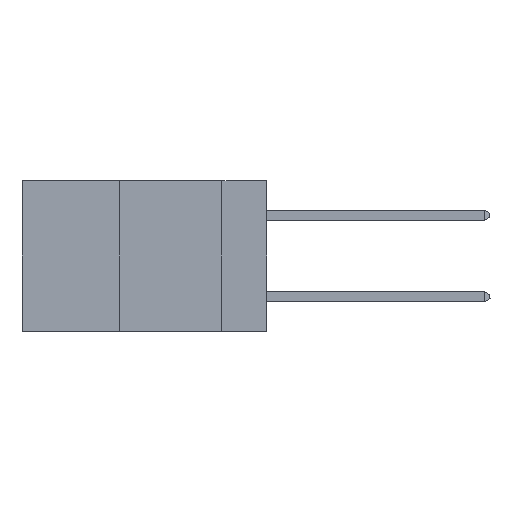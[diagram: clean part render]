
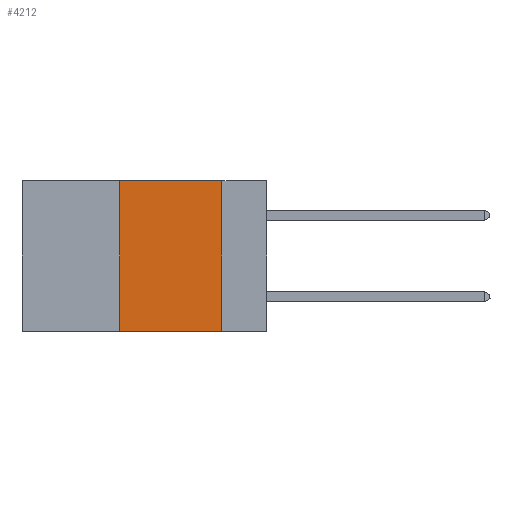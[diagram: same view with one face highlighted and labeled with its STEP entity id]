
A CAD part, left-side view. The second image highlights one B-rep face of the part: STEP entity #4212.
In plain terms, the highlighted planar face has unit normal (-1, 0, 0).
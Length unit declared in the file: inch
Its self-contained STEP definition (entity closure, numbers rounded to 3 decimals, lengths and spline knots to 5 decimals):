
#43 = DIRECTION ( 'NONE',  ( 0., 0., -1. ) ) ;
#694 = EDGE_CURVE ( 'NONE', #19665, #8763, #22387, .T. ) ;
#1122 = EDGE_LOOP ( 'NONE', ( #20354, #18112, #22234, #12950 ) ) ;
#1614 = VECTOR ( 'NONE', #10690, 39.37008 ) ;
#1922 = AXIS2_PLACEMENT_3D ( 'NONE', #17055, #19827, #19886 ) ;
#2214 = DIRECTION ( 'NONE',  ( 0., -1., 0. ) ) ;
#2495 = LINE ( 'NONE', #20569, #10209 ) ;
#2637 = VECTOR ( 'NONE', #43, 39.37008 ) ;
#4154 = EDGE_CURVE ( 'NONE', #19665, #20571, #2495, .T. ) ;
#4212 = ADVANCED_FACE ( 'NONE', ( #9643 ), #4715, .F. ) ;
#4715 = PLANE ( 'NONE',  #1922 ) ;
#5389 = LINE ( 'NONE', #10596, #2637 ) ;
#5677 = CARTESIAN_POINT ( 'NONE',  ( 0., 0.6, -0.37 ) ) ;
#5938 = VERTEX_POINT ( 'NONE', #14567 ) ;
#8763 = VERTEX_POINT ( 'NONE', #19301 ) ;
#9643 = FACE_OUTER_BOUND ( 'NONE', #1122, .T. ) ;
#10209 = VECTOR ( 'NONE', #13452, 39.37008 ) ;
#10596 = CARTESIAN_POINT ( 'NONE',  ( 0., 0.11, 0. ) ) ;
#10690 = DIRECTION ( 'NONE',  ( 0., -1., 0. ) ) ;
#10923 = LINE ( 'NONE', #21168, #1614 ) ;
#12950 = ORIENTED_EDGE ( 'NONE', *, *, #694, .T. ) ;
#13452 = DIRECTION ( 'NONE',  ( 0., 0., 1. ) ) ;
#14567 = CARTESIAN_POINT ( 'NONE',  ( 0., 0.11, 0. ) ) ;
#16491 = EDGE_CURVE ( 'NONE', #20571, #5938, #10923, .T. ) ;
#17055 = CARTESIAN_POINT ( 'NONE',  ( 0., 0.6, 0. ) ) ;
#17734 = VECTOR ( 'NONE', #2214, 39.37008 ) ;
#18112 = ORIENTED_EDGE ( 'NONE', *, *, #16491, .F. ) ;
#18362 = EDGE_CURVE ( 'NONE', #5938, #8763, #5389, .T. ) ;
#18800 = CARTESIAN_POINT ( 'NONE',  ( 0., 0.36, 0. ) ) ;
#19188 = CARTESIAN_POINT ( 'NONE',  ( 0., 0.36, -0.37 ) ) ;
#19301 = CARTESIAN_POINT ( 'NONE',  ( 0., 0.11, -0.37 ) ) ;
#19665 = VERTEX_POINT ( 'NONE', #19188 ) ;
#19827 = DIRECTION ( 'NONE',  ( 1., 0., 0. ) ) ;
#19886 = DIRECTION ( 'NONE',  ( 0., 0., -1. ) ) ;
#20354 = ORIENTED_EDGE ( 'NONE', *, *, #18362, .F. ) ;
#20569 = CARTESIAN_POINT ( 'NONE',  ( 0., 0.36, 0. ) ) ;
#20571 = VERTEX_POINT ( 'NONE', #18800 ) ;
#21168 = CARTESIAN_POINT ( 'NONE',  ( 0., 0.6, 0. ) ) ;
#22234 = ORIENTED_EDGE ( 'NONE', *, *, #4154, .F. ) ;
#22387 = LINE ( 'NONE', #5677, #17734 ) ;
